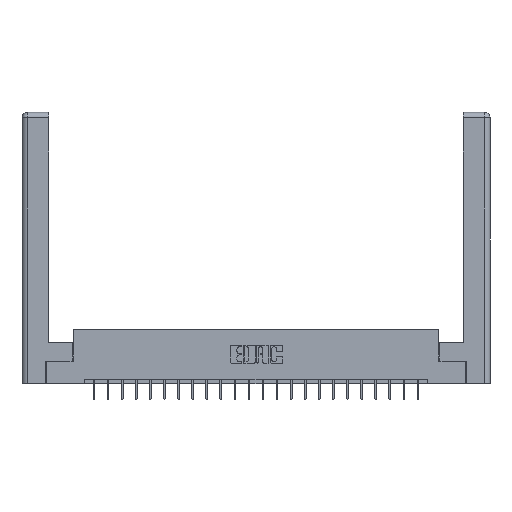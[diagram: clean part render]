
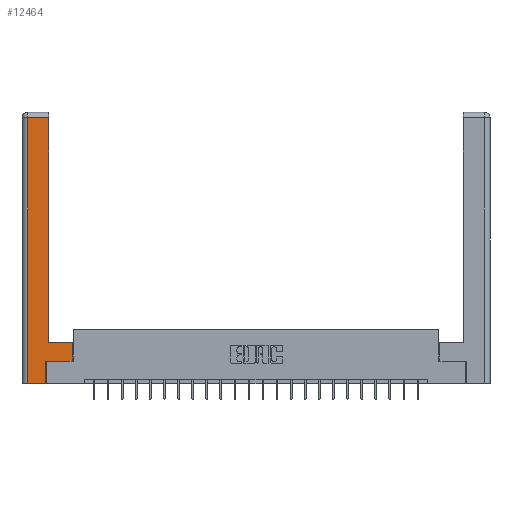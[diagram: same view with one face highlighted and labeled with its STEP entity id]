
A CAD part, top view. The second image highlights one B-rep face of the part: STEP entity #12464.
In plain terms, the highlighted planar face has unit normal (0, 0, 1).
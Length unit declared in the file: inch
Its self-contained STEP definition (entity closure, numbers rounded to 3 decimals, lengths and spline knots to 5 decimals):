
#310 = AXIS2_PLACEMENT_3D ( 'NONE', #17203, #11671, #2641 ) ;
#565 = LINE ( 'NONE', #6739, #14243 ) ;
#1497 = ORIENTED_EDGE ( 'NONE', *, *, #11982, .T. ) ;
#1658 = VECTOR ( 'NONE', #10475, 39.37008 ) ;
#2014 = VERTEX_POINT ( 'NONE', #3586 ) ;
#2311 = VERTEX_POINT ( 'NONE', #22383 ) ;
#2641 = DIRECTION ( 'NONE',  ( -1., 0., 0. ) ) ;
#2712 = VERTEX_POINT ( 'NONE', #6803 ) ;
#3345 = CARTESIAN_POINT ( 'NONE',  ( 0.565, 0.45, 0. ) ) ;
#3359 = LINE ( 'NONE', #8371, #20205 ) ;
#3453 = CARTESIAN_POINT ( 'NONE',  ( 0.565, 0.45, 0. ) ) ;
#3486 = CARTESIAN_POINT ( 'NONE',  ( 0.295, 0.45, 0. ) ) ;
#3550 = VERTEX_POINT ( 'NONE', #3345 ) ;
#3586 = CARTESIAN_POINT ( 'NONE',  ( 0.265, 0.245, 0. ) ) ;
#4123 = CARTESIAN_POINT ( 'NONE',  ( 0.0615, 0., 0. ) ) ;
#4670 = CARTESIAN_POINT ( 'NONE',  ( 0.0615, 2.94, 0. ) ) ;
#4807 = CARTESIAN_POINT ( 'NONE',  ( 0.265, 0.245, 0. ) ) ;
#6248 = ORIENTED_EDGE ( 'NONE', *, *, #18269, .T. ) ;
#6739 = CARTESIAN_POINT ( 'NONE',  ( 0.0615, 2.94, 0. ) ) ;
#6803 = CARTESIAN_POINT ( 'NONE',  ( 0.265, 0., 0. ) ) ;
#7296 = DIRECTION ( 'NONE',  ( -1., 0., 0. ) ) ;
#7341 = ORIENTED_EDGE ( 'NONE', *, *, #19990, .T. ) ;
#8275 = EDGE_CURVE ( 'NONE', #2712, #2014, #17931, .T. ) ;
#8371 = CARTESIAN_POINT ( 'NONE',  ( 0.295, 3., 0. ) ) ;
#8391 = LINE ( 'NONE', #16299, #8966 ) ;
#8928 = VECTOR ( 'NONE', #12579, 39.37008 ) ;
#8950 = VERTEX_POINT ( 'NONE', #9992 ) ;
#8966 = VECTOR ( 'NONE', #16378, 39.37008 ) ;
#9053 = CARTESIAN_POINT ( 'NONE',  ( 0.0615, 0., 0. ) ) ;
#9670 = VERTEX_POINT ( 'NONE', #4670 ) ;
#9805 = EDGE_CURVE ( 'NONE', #9670, #20546, #20720, .T. ) ;
#9992 = CARTESIAN_POINT ( 'NONE',  ( 0.565, 0.245, 0. ) ) ;
#10475 = DIRECTION ( 'NONE',  ( 0., 1., 0. ) ) ;
#10718 = VECTOR ( 'NONE', #21653, 39.37008 ) ;
#10996 = VERTEX_POINT ( 'NONE', #3486 ) ;
#11003 = DIRECTION ( 'NONE',  ( -1., 0., 0. ) ) ;
#11238 = VECTOR ( 'NONE', #11003, 39.37008 ) ;
#11671 = DIRECTION ( 'NONE',  ( 0., 0., -1. ) ) ;
#11982 = EDGE_CURVE ( 'NONE', #20546, #2712, #13110, .T. ) ;
#12035 = LINE ( 'NONE', #22128, #11238 ) ;
#12155 = EDGE_CURVE ( 'NONE', #2311, #9670, #565, .T. ) ;
#12464 = ADVANCED_FACE ( 'NONE', ( #12471 ), #17125, .F. ) ;
#12471 = FACE_OUTER_BOUND ( 'NONE', #21255, .T. ) ;
#12579 = DIRECTION ( 'NONE',  ( 0., 1., 0. ) ) ;
#13110 = LINE ( 'NONE', #13896, #13708 ) ;
#13238 = LINE ( 'NONE', #3453, #8928 ) ;
#13708 = VECTOR ( 'NONE', #15430, 39.37008 ) ;
#13896 = CARTESIAN_POINT ( 'NONE',  ( 0.265, 0., 0. ) ) ;
#13966 = DIRECTION ( 'NONE',  ( 0., 1., 0. ) ) ;
#14243 = VECTOR ( 'NONE', #7296, 39.37008 ) ;
#15430 = DIRECTION ( 'NONE',  ( 1., 0., 0. ) ) ;
#15529 = ORIENTED_EDGE ( 'NONE', *, *, #12155, .T. ) ;
#16172 = ORIENTED_EDGE ( 'NONE', *, *, #19438, .T. ) ;
#16299 = CARTESIAN_POINT ( 'NONE',  ( 0.565, 0.245, 0. ) ) ;
#16378 = DIRECTION ( 'NONE',  ( 1., 0., 0. ) ) ;
#17125 = PLANE ( 'NONE',  #310 ) ;
#17203 = CARTESIAN_POINT ( 'NONE',  ( 0., 0., 0. ) ) ;
#17931 = LINE ( 'NONE', #4807, #1658 ) ;
#18269 = EDGE_CURVE ( 'NONE', #2014, #8950, #8391, .T. ) ;
#19438 = EDGE_CURVE ( 'NONE', #8950, #3550, #13238, .T. ) ;
#19990 = EDGE_CURVE ( 'NONE', #10996, #2311, #3359, .T. ) ;
#20205 = VECTOR ( 'NONE', #13966, 39.37008 ) ;
#20464 = ORIENTED_EDGE ( 'NONE', *, *, #9805, .T. ) ;
#20546 = VERTEX_POINT ( 'NONE', #4123 ) ;
#20719 = ORIENTED_EDGE ( 'NONE', *, *, #21778, .T. ) ;
#20720 = LINE ( 'NONE', #9053, #10718 ) ;
#21255 = EDGE_LOOP ( 'NONE', ( #7341, #15529, #20464, #1497, #21874, #6248, #16172, #20719 ) ) ;
#21653 = DIRECTION ( 'NONE',  ( 0., -1., 0. ) ) ;
#21778 = EDGE_CURVE ( 'NONE', #3550, #10996, #12035, .T. ) ;
#21874 = ORIENTED_EDGE ( 'NONE', *, *, #8275, .T. ) ;
#22128 = CARTESIAN_POINT ( 'NONE',  ( 0.295, 0.45, 0. ) ) ;
#22383 = CARTESIAN_POINT ( 'NONE',  ( 0.295, 2.94, 0. ) ) ;
